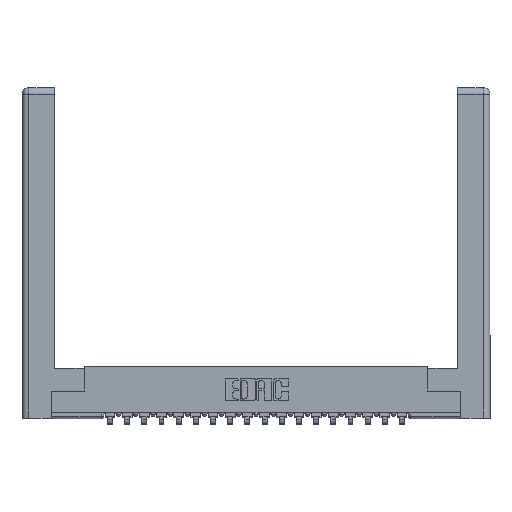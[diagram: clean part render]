
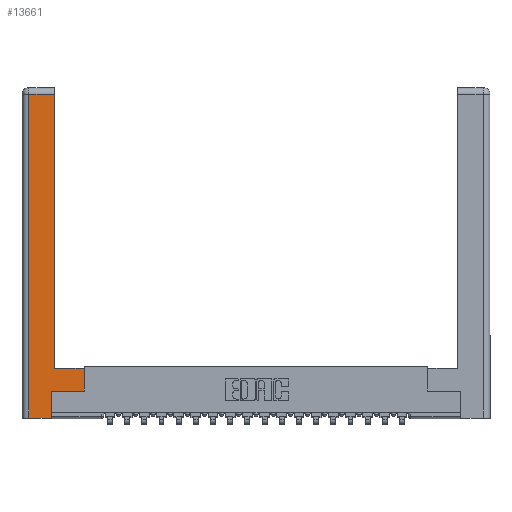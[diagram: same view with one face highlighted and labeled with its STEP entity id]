
A CAD part, top view. The second image highlights one B-rep face of the part: STEP entity #13661.
In plain terms, the highlighted planar face has unit normal (0, 0, 1).
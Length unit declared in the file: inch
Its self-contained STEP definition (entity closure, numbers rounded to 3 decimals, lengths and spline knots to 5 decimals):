
#225 = DIRECTION ( 'NONE',  ( 0., 1., 0. ) ) ;
#521 = EDGE_CURVE ( 'NONE', #10320, #1969, #21069, .T. ) ;
#1131 = CARTESIAN_POINT ( 'NONE',  ( 0.295, 2.94, 0. ) ) ;
#1787 = CARTESIAN_POINT ( 'NONE',  ( 0.295, 3., 0. ) ) ;
#1969 = VERTEX_POINT ( 'NONE', #15852 ) ;
#2071 = CARTESIAN_POINT ( 'NONE',  ( 0.565, 0.45, 0. ) ) ;
#2547 = CARTESIAN_POINT ( 'NONE',  ( 0., 0., 0. ) ) ;
#2638 = VECTOR ( 'NONE', #10334, 39.37008 ) ;
#2849 = EDGE_CURVE ( 'NONE', #17342, #14397, #10391, .T. ) ;
#3152 = VERTEX_POINT ( 'NONE', #16973 ) ;
#3238 = VECTOR ( 'NONE', #17230, 39.37008 ) ;
#3298 = LINE ( 'NONE', #2071, #14281 ) ;
#3953 = VERTEX_POINT ( 'NONE', #1131 ) ;
#4505 = CARTESIAN_POINT ( 'NONE',  ( 0.265, 0., 0. ) ) ;
#4983 = VECTOR ( 'NONE', #12442, 39.37008 ) ;
#5194 = CARTESIAN_POINT ( 'NONE',  ( 0.265, 0., 0. ) ) ;
#5261 = EDGE_LOOP ( 'NONE', ( #16454, #11981, #12685, #10925, #12949, #10017, #14416, #19656 ) ) ;
#5406 = LINE ( 'NONE', #18783, #3238 ) ;
#5923 = CARTESIAN_POINT ( 'NONE',  ( 0.565, 0.245, 0. ) ) ;
#6035 = CARTESIAN_POINT ( 'NONE',  ( 0.0615, 0., 0. ) ) ;
#6200 = EDGE_CURVE ( 'NONE', #1969, #17342, #3298, .T. ) ;
#6258 = CARTESIAN_POINT ( 'NONE',  ( 0.565, 0.45, 0. ) ) ;
#8621 = VECTOR ( 'NONE', #21766, 39.37008 ) ;
#8828 = DIRECTION ( 'NONE',  ( -1., 0., 0. ) ) ;
#8930 = DIRECTION ( 'NONE',  ( 0., 1., 0. ) ) ;
#9074 = DIRECTION ( 'NONE',  ( 0., 0., -1. ) ) ;
#9426 = CARTESIAN_POINT ( 'NONE',  ( 0.0615, 0., 0. ) ) ;
#9914 = LINE ( 'NONE', #4505, #8621 ) ;
#10017 = ORIENTED_EDGE ( 'NONE', *, *, #521, .T. ) ;
#10310 = LINE ( 'NONE', #1787, #21667 ) ;
#10320 = VERTEX_POINT ( 'NONE', #12214 ) ;
#10334 = DIRECTION ( 'NONE',  ( 0., 1., 0. ) ) ;
#10391 = LINE ( 'NONE', #18565, #11137 ) ;
#10633 = FACE_OUTER_BOUND ( 'NONE', #5261, .T. ) ;
#10925 = ORIENTED_EDGE ( 'NONE', *, *, #16905, .T. ) ;
#11137 = VECTOR ( 'NONE', #8828, 39.37008 ) ;
#11801 = CARTESIAN_POINT ( 'NONE',  ( 0.295, 0.45, 0. ) ) ;
#11981 = ORIENTED_EDGE ( 'NONE', *, *, #19789, .T. ) ;
#12214 = CARTESIAN_POINT ( 'NONE',  ( 0.265, 0.245, 0. ) ) ;
#12442 = DIRECTION ( 'NONE',  ( 0., -1., 0. ) ) ;
#12685 = ORIENTED_EDGE ( 'NONE', *, *, #20429, .T. ) ;
#12949 = ORIENTED_EDGE ( 'NONE', *, *, #16188, .T. ) ;
#13661 = ADVANCED_FACE ( 'NONE', ( #10633 ), #19374, .F. ) ;
#13948 = VERTEX_POINT ( 'NONE', #5194 ) ;
#14281 = VECTOR ( 'NONE', #8930, 39.37008 ) ;
#14397 = VERTEX_POINT ( 'NONE', #11801 ) ;
#14416 = ORIENTED_EDGE ( 'NONE', *, *, #6200, .T. ) ;
#14531 = AXIS2_PLACEMENT_3D ( 'NONE', #2547, #9074, #16048 ) ;
#14774 = EDGE_CURVE ( 'NONE', #14397, #3953, #10310, .T. ) ;
#15852 = CARTESIAN_POINT ( 'NONE',  ( 0.565, 0.245, 0. ) ) ;
#16048 = DIRECTION ( 'NONE',  ( -1., 0., 0. ) ) ;
#16188 = EDGE_CURVE ( 'NONE', #13948, #10320, #18401, .T. ) ;
#16454 = ORIENTED_EDGE ( 'NONE', *, *, #14774, .T. ) ;
#16905 = EDGE_CURVE ( 'NONE', #17781, #13948, #9914, .T. ) ;
#16973 = CARTESIAN_POINT ( 'NONE',  ( 0.0615, 2.94, 0. ) ) ;
#17230 = DIRECTION ( 'NONE',  ( -1., 0., 0. ) ) ;
#17342 = VERTEX_POINT ( 'NONE', #6258 ) ;
#17781 = VERTEX_POINT ( 'NONE', #9426 ) ;
#18401 = LINE ( 'NONE', #18734, #2638 ) ;
#18565 = CARTESIAN_POINT ( 'NONE',  ( 0.295, 0.45, 0. ) ) ;
#18734 = CARTESIAN_POINT ( 'NONE',  ( 0.265, 0.245, 0. ) ) ;
#18783 = CARTESIAN_POINT ( 'NONE',  ( 0.0615, 2.94, 0. ) ) ;
#19374 = PLANE ( 'NONE',  #14531 ) ;
#19419 = DIRECTION ( 'NONE',  ( 1., 0., 0. ) ) ;
#19656 = ORIENTED_EDGE ( 'NONE', *, *, #2849, .T. ) ;
#19697 = VECTOR ( 'NONE', #19419, 39.37008 ) ;
#19789 = EDGE_CURVE ( 'NONE', #3953, #3152, #5406, .T. ) ;
#20429 = EDGE_CURVE ( 'NONE', #3152, #17781, #21174, .T. ) ;
#21069 = LINE ( 'NONE', #5923, #19697 ) ;
#21174 = LINE ( 'NONE', #6035, #4983 ) ;
#21667 = VECTOR ( 'NONE', #225, 39.37008 ) ;
#21766 = DIRECTION ( 'NONE',  ( 1., 0., 0. ) ) ;
